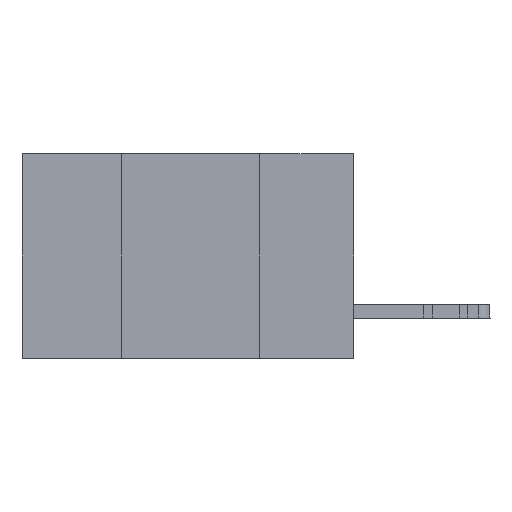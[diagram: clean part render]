
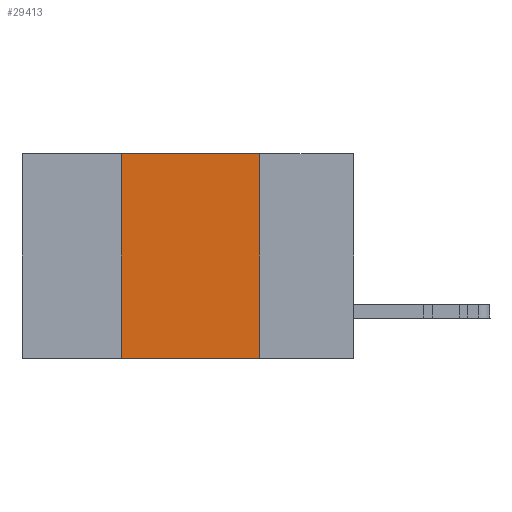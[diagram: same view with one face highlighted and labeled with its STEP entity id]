
A CAD part, left-side view. The second image highlights one B-rep face of the part: STEP entity #29413.
In plain terms, the highlighted planar face has unit normal (-1, 0, 0).
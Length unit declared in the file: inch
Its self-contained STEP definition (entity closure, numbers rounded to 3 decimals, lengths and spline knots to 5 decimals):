
#1529 = CARTESIAN_POINT ( 'NONE',  ( 0., 0.42, -0.37 ) ) ;
#2304 = EDGE_LOOP ( 'NONE', ( #17496, #23070, #44078, #6696 ) ) ;
#3157 = VECTOR ( 'NONE', #39644, 39.37008 ) ;
#4121 = VERTEX_POINT ( 'NONE', #18601 ) ;
#6073 = DIRECTION ( 'NONE',  ( 0., -1., 0. ) ) ;
#6696 = ORIENTED_EDGE ( 'NONE', *, *, #18242, .T. ) ;
#12748 = CARTESIAN_POINT ( 'NONE',  ( 0., 0.6, -0.37 ) ) ;
#16262 = LINE ( 'NONE', #12748, #3157 ) ;
#16536 = DIRECTION ( 'NONE',  ( 0., 0., -1. ) ) ;
#17496 = ORIENTED_EDGE ( 'NONE', *, *, #39290, .F. ) ;
#18242 = EDGE_CURVE ( 'NONE', #34178, #25626, #16262, .T. ) ;
#18601 = CARTESIAN_POINT ( 'NONE',  ( 0., 0.17, 0. ) ) ;
#19035 = LINE ( 'NONE', #44106, #32215 ) ;
#19261 = EDGE_CURVE ( 'NONE', #34178, #20673, #26297, .T. ) ;
#19414 = LINE ( 'NONE', #31967, #29019 ) ;
#20673 = VERTEX_POINT ( 'NONE', #29983 ) ;
#22712 = DIRECTION ( 'NONE',  ( 0., 0., -1. ) ) ;
#23070 = ORIENTED_EDGE ( 'NONE', *, *, #48760, .F. ) ;
#25626 = VERTEX_POINT ( 'NONE', #26212 ) ;
#26212 = CARTESIAN_POINT ( 'NONE',  ( 0., 0.17, -0.37 ) ) ;
#26297 = LINE ( 'NONE', #38059, #27493 ) ;
#27493 = VECTOR ( 'NONE', #42203, 39.37008 ) ;
#29019 = VECTOR ( 'NONE', #16536, 39.37008 ) ;
#29413 = ADVANCED_FACE ( 'NONE', ( #31269 ), #42220, .F. ) ;
#29983 = CARTESIAN_POINT ( 'NONE',  ( 0., 0.42, 0. ) ) ;
#30270 = CARTESIAN_POINT ( 'NONE',  ( 0., 0.6, 0. ) ) ;
#31269 = FACE_OUTER_BOUND ( 'NONE', #2304, .T. ) ;
#31967 = CARTESIAN_POINT ( 'NONE',  ( 0., 0.17, 0. ) ) ;
#32215 = VECTOR ( 'NONE', #6073, 39.37008 ) ;
#32820 = AXIS2_PLACEMENT_3D ( 'NONE', #30270, #38562, #22712 ) ;
#34178 = VERTEX_POINT ( 'NONE', #1529 ) ;
#38059 = CARTESIAN_POINT ( 'NONE',  ( 0., 0.42, 0. ) ) ;
#38562 = DIRECTION ( 'NONE',  ( 1., 0., 0. ) ) ;
#39290 = EDGE_CURVE ( 'NONE', #4121, #25626, #19414, .T. ) ;
#39644 = DIRECTION ( 'NONE',  ( 0., -1., 0. ) ) ;
#42203 = DIRECTION ( 'NONE',  ( 0., 0., 1. ) ) ;
#42220 = PLANE ( 'NONE',  #32820 ) ;
#44078 = ORIENTED_EDGE ( 'NONE', *, *, #19261, .F. ) ;
#44106 = CARTESIAN_POINT ( 'NONE',  ( 0., 0.6, 0. ) ) ;
#48760 = EDGE_CURVE ( 'NONE', #20673, #4121, #19035, .T. ) ;
